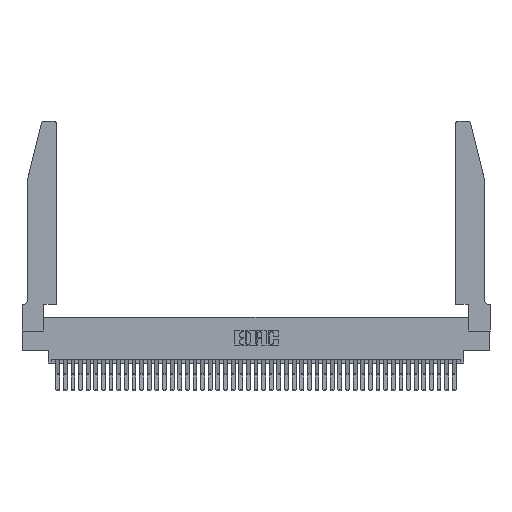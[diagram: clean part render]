
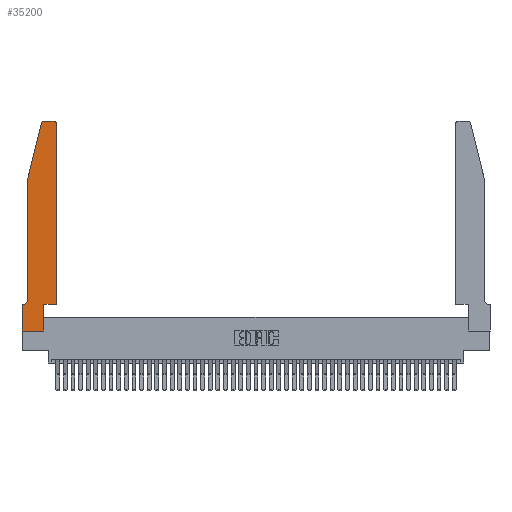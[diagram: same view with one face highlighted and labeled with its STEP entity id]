
A CAD part, top view. The second image highlights one B-rep face of the part: STEP entity #35200.
In plain terms, the highlighted planar face has unit normal (0, 0, 1).
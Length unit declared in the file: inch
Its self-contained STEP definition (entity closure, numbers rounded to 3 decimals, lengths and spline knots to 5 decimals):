
#1193 = ORIENTED_EDGE ( 'NONE', *, *, #22711, .T. ) ;
#1353 = CARTESIAN_POINT ( 'NONE',  ( 0.4205, 2.72, 0.37 ) ) ;
#1399 = EDGE_CURVE ( 'NONE', #24224, #19705, #3679, .T. ) ;
#1406 = DIRECTION ( 'NONE',  ( 1., 0., 0. ) ) ;
#1732 = CARTESIAN_POINT ( 'NONE',  ( 0., 0., 0.37 ) ) ;
#2397 = LINE ( 'NONE', #44159, #38341 ) ;
#2899 = VECTOR ( 'NONE', #28804, 39.37008 ) ;
#3015 = CARTESIAN_POINT ( 'NONE',  ( 0.2865, 0., 0.37 ) ) ;
#3259 = DIRECTION ( 'NONE',  ( 0., -1., 0. ) ) ;
#3504 = VERTEX_POINT ( 'NONE', #1732 ) ;
#3679 = LINE ( 'NONE', #10928, #38520 ) ;
#3686 = CARTESIAN_POINT ( 'NONE',  ( 0.0055, 0.35, 0.37 ) ) ;
#4349 = AXIS2_PLACEMENT_3D ( 'NONE', #36921, #16108, #40412 ) ;
#4392 = CARTESIAN_POINT ( 'NONE',  ( 0., 0., 0.37 ) ) ;
#4425 = VERTEX_POINT ( 'NONE', #36137 ) ;
#4861 = DIRECTION ( 'NONE',  ( 1., 0., 0. ) ) ;
#5078 = ORIENTED_EDGE ( 'NONE', *, *, #10028, .T. ) ;
#5517 = CARTESIAN_POINT ( 'NONE',  ( 0.4505, 0.35, 0.37 ) ) ;
#6141 = DIRECTION ( 'NONE',  ( 0., 1., 0. ) ) ;
#6147 = ORIENTED_EDGE ( 'NONE', *, *, #27109, .T. ) ;
#6609 = VERTEX_POINT ( 'NONE', #36421 ) ;
#7772 = VECTOR ( 'NONE', #33463, 39.37008 ) ;
#7821 = ORIENTED_EDGE ( 'NONE', *, *, #1399, .T. ) ;
#7839 = VERTEX_POINT ( 'NONE', #35544 ) ;
#9188 = LINE ( 'NONE', #5517, #36951 ) ;
#9722 = CARTESIAN_POINT ( 'NONE',  ( 0., 0.35, 0.37 ) ) ;
#10028 = EDGE_CURVE ( 'NONE', #3504, #32432, #40218, .T. ) ;
#10214 = VECTOR ( 'NONE', #3259, 39.37008 ) ;
#10928 = CARTESIAN_POINT ( 'NONE',  ( 0.0755, 0.35, 0.37 ) ) ;
#11088 = LINE ( 'NONE', #4392, #2899 ) ;
#11223 = CARTESIAN_POINT ( 'NONE',  ( 0., 0.35, 0.37 ) ) ;
#11465 = CIRCLE ( 'NONE', #26576, 0.03 ) ;
#12248 = VECTOR ( 'NONE', #32461, 39.37008 ) ;
#12495 = VERTEX_POINT ( 'NONE', #21882 ) ;
#13003 = DIRECTION ( 'NONE',  ( -1., 0., 0. ) ) ;
#13175 = EDGE_CURVE ( 'NONE', #19705, #3504, #11088, .T. ) ;
#13492 = EDGE_CURVE ( 'NONE', #38294, #24224, #29084, .T. ) ;
#13564 = VECTOR ( 'NONE', #42297, 39.37008 ) ;
#14116 = EDGE_CURVE ( 'NONE', #32432, #4425, #37574, .T. ) ;
#14477 = CARTESIAN_POINT ( 'NONE',  ( 0., 0., 0.37 ) ) ;
#15995 = CARTESIAN_POINT ( 'NONE',  ( 0.4505, 0.35, 0.37 ) ) ;
#16047 = DIRECTION ( 'NONE',  ( 1., 0., 0. ) ) ;
#16108 = DIRECTION ( 'NONE',  ( 0., 0., -1. ) ) ;
#17039 = LINE ( 'NONE', #15995, #7772 ) ;
#17463 = AXIS2_PLACEMENT_3D ( 'NONE', #11223, #18441, #42685 ) ;
#17979 = DIRECTION ( 'NONE',  ( -1., 0., 0. ) ) ;
#18441 = DIRECTION ( 'NONE',  ( 0., 0., 1. ) ) ;
#18514 = EDGE_CURVE ( 'NONE', #24774, #12495, #2397, .T. ) ;
#18763 = ORIENTED_EDGE ( 'NONE', *, *, #13492, .T. ) ;
#19377 = ORIENTED_EDGE ( 'NONE', *, *, #24723, .T. ) ;
#19705 = VERTEX_POINT ( 'NONE', #9722 ) ;
#21347 = VECTOR ( 'NONE', #6141, 39.37008 ) ;
#21478 = ORIENTED_EDGE ( 'NONE', *, *, #23747, .T. ) ;
#21802 = PLANE ( 'NONE',  #17463 ) ;
#21882 = CARTESIAN_POINT ( 'NONE',  ( 0.284, 2.75, 0.37 ) ) ;
#22375 = DIRECTION ( 'NONE',  ( 0., 0., 1. ) ) ;
#22711 = EDGE_CURVE ( 'NONE', #24355, #30467, #17039, .T. ) ;
#23559 = CARTESIAN_POINT ( 'NONE',  ( 0.2865, 0.35, 0.37 ) ) ;
#23747 = EDGE_CURVE ( 'NONE', #12495, #6609, #11465, .T. ) ;
#24224 = VERTEX_POINT ( 'NONE', #3686 ) ;
#24355 = VERTEX_POINT ( 'NONE', #28158 ) ;
#24723 = EDGE_CURVE ( 'NONE', #4425, #24355, #9188, .T. ) ;
#24774 = VERTEX_POINT ( 'NONE', #43843 ) ;
#25809 = DIRECTION ( 'NONE',  ( 0., 0., 1. ) ) ;
#26308 = EDGE_CURVE ( 'NONE', #7839, #38294, #37968, .T. ) ;
#26576 = AXIS2_PLACEMENT_3D ( 'NONE', #43110, #22375, #1406 ) ;
#27109 = EDGE_CURVE ( 'NONE', #6609, #7839, #41091, .T. ) ;
#27565 = EDGE_CURVE ( 'NONE', #30467, #24774, #41049, .T. ) ;
#28158 = CARTESIAN_POINT ( 'NONE',  ( 0.4505, 0.35, 0.37 ) ) ;
#28804 = DIRECTION ( 'NONE',  ( 0., -1., 0. ) ) ;
#29050 = ORIENTED_EDGE ( 'NONE', *, *, #27565, .T. ) ;
#29084 = CIRCLE ( 'NONE', #4349, 0.07 ) ;
#29134 = ORIENTED_EDGE ( 'NONE', *, *, #18514, .T. ) ;
#29645 = ORIENTED_EDGE ( 'NONE', *, *, #13175, .T. ) ;
#29879 = EDGE_LOOP ( 'NONE', ( #29134, #21478, #6147, #43158, #18763, #7821, #29645, #5078, #31309, #19377, #1193, #29050 ) ) ;
#30467 = VERTEX_POINT ( 'NONE', #33925 ) ;
#31309 = ORIENTED_EDGE ( 'NONE', *, *, #14116, .T. ) ;
#32432 = VERTEX_POINT ( 'NONE', #3015 ) ;
#32461 = DIRECTION ( 'NONE',  ( -0.239, -0.971, 0. ) ) ;
#33463 = DIRECTION ( 'NONE',  ( 0., 1., 0. ) ) ;
#33925 = CARTESIAN_POINT ( 'NONE',  ( 0.4505, 2.72, 0.37 ) ) ;
#34155 = AXIS2_PLACEMENT_3D ( 'NONE', #1353, #25809, #4861 ) ;
#35200 = ADVANCED_FACE ( 'NONE', ( #40599 ), #21802, .T. ) ;
#35544 = CARTESIAN_POINT ( 'NONE',  ( 0.0755, 2., 0.37 ) ) ;
#35784 = CARTESIAN_POINT ( 'NONE',  ( 0.0755, 2., 0.37 ) ) ;
#36137 = CARTESIAN_POINT ( 'NONE',  ( 0.2865, 0.35, 0.37 ) ) ;
#36421 = CARTESIAN_POINT ( 'NONE',  ( 0.25487, 2.72718, 0.37 ) ) ;
#36921 = CARTESIAN_POINT ( 'NONE',  ( 0.0055, 0.42, 0.37 ) ) ;
#36951 = VECTOR ( 'NONE', #16047, 39.37008 ) ;
#37574 = LINE ( 'NONE', #23559, #21347 ) ;
#37968 = LINE ( 'NONE', #44939, #10214 ) ;
#38294 = VERTEX_POINT ( 'NONE', #43592 ) ;
#38341 = VECTOR ( 'NONE', #13003, 39.37008 ) ;
#38520 = VECTOR ( 'NONE', #17979, 39.37008 ) ;
#40218 = LINE ( 'NONE', #14477, #13564 ) ;
#40412 = DIRECTION ( 'NONE',  ( -1., 0., 0. ) ) ;
#40599 = FACE_OUTER_BOUND ( 'NONE', #29879, .T. ) ;
#41049 = CIRCLE ( 'NONE', #34155, 0.03 ) ;
#41091 = LINE ( 'NONE', #35784, #12248 ) ;
#42297 = DIRECTION ( 'NONE',  ( 1., 0., 0. ) ) ;
#42685 = DIRECTION ( 'NONE',  ( 1., 0., 0. ) ) ;
#43110 = CARTESIAN_POINT ( 'NONE',  ( 0.284, 2.72, 0.37 ) ) ;
#43158 = ORIENTED_EDGE ( 'NONE', *, *, #26308, .T. ) ;
#43592 = CARTESIAN_POINT ( 'NONE',  ( 0.0755, 0.42, 0.37 ) ) ;
#43843 = CARTESIAN_POINT ( 'NONE',  ( 0.4205, 2.75, 0.37 ) ) ;
#44159 = CARTESIAN_POINT ( 'NONE',  ( 0.2605, 2.75, 0.37 ) ) ;
#44939 = CARTESIAN_POINT ( 'NONE',  ( 0.0755, 2., 0.37 ) ) ;
